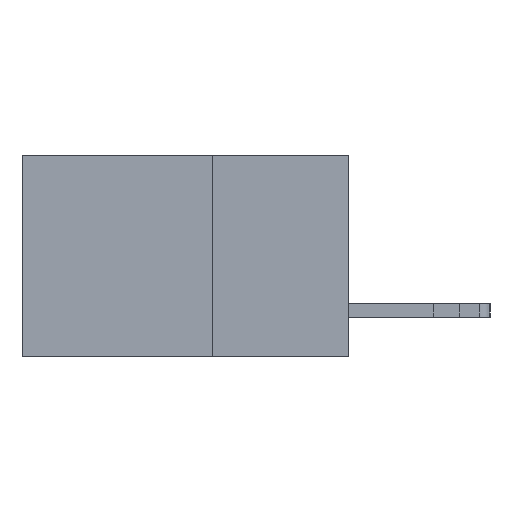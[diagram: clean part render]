
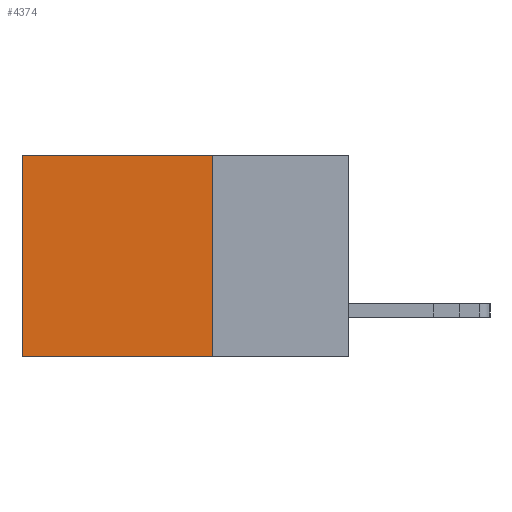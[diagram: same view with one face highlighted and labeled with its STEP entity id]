
A CAD part, left-side view. The second image highlights one B-rep face of the part: STEP entity #4374.
In plain terms, the highlighted planar face has unit normal (-1, 0, 0).
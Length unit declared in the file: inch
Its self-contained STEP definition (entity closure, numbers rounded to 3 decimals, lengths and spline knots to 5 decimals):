
#1281 = LINE ( 'NONE', #13152, #12820 ) ;
#1387 = DIRECTION ( 'NONE',  ( 0., 0., -1. ) ) ;
#1881 = VECTOR ( 'NONE', #18855, 39.37008 ) ;
#2364 = LINE ( 'NONE', #11405, #1881 ) ;
#2693 = VERTEX_POINT ( 'NONE', #4272 ) ;
#2909 = CARTESIAN_POINT ( 'NONE',  ( 0.298, 0.25, 0. ) ) ;
#4272 = CARTESIAN_POINT ( 'NONE',  ( 0.298, 0.25, -0.37 ) ) ;
#4374 = ADVANCED_FACE ( 'NONE', ( #13773 ), #11928, .F. ) ;
#4414 = DIRECTION ( 'NONE',  ( 1., 0., 0. ) ) ;
#4435 = EDGE_LOOP ( 'NONE', ( #9467, #10692, #15013, #9025 ) ) ;
#4733 = EDGE_CURVE ( 'NONE', #7990, #11289, #11190, .T. ) ;
#4887 = EDGE_CURVE ( 'NONE', #10564, #7990, #1281, .T. ) ;
#5282 = LINE ( 'NONE', #10419, #16817 ) ;
#7990 = VERTEX_POINT ( 'NONE', #11237 ) ;
#9025 = ORIENTED_EDGE ( 'NONE', *, *, #4887, .T. ) ;
#9467 = ORIENTED_EDGE ( 'NONE', *, *, #4733, .T. ) ;
#9555 = CARTESIAN_POINT ( 'NONE',  ( 0.298, 0.25, 0. ) ) ;
#9861 = DIRECTION ( 'NONE',  ( 0., 0., -1. ) ) ;
#10419 = CARTESIAN_POINT ( 'NONE',  ( 0.298, 0.25, 0. ) ) ;
#10564 = VERTEX_POINT ( 'NONE', #9555 ) ;
#10692 = ORIENTED_EDGE ( 'NONE', *, *, #18656, .F. ) ;
#11190 = LINE ( 'NONE', #14215, #14708 ) ;
#11237 = CARTESIAN_POINT ( 'NONE',  ( 0.298, 0.6, 0. ) ) ;
#11289 = VERTEX_POINT ( 'NONE', #18541 ) ;
#11405 = CARTESIAN_POINT ( 'NONE',  ( 0.298, 0.25, -0.37 ) ) ;
#11928 = PLANE ( 'NONE',  #13498 ) ;
#12820 = VECTOR ( 'NONE', #16102, 39.37008 ) ;
#13152 = CARTESIAN_POINT ( 'NONE',  ( 0.298, 0.25, 0. ) ) ;
#13498 = AXIS2_PLACEMENT_3D ( 'NONE', #2909, #4414, #14943 ) ;
#13773 = FACE_OUTER_BOUND ( 'NONE', #4435, .T. ) ;
#14215 = CARTESIAN_POINT ( 'NONE',  ( 0.298, 0.6, 0. ) ) ;
#14708 = VECTOR ( 'NONE', #9861, 39.37008 ) ;
#14943 = DIRECTION ( 'NONE',  ( 0., 0., -1. ) ) ;
#15013 = ORIENTED_EDGE ( 'NONE', *, *, #16574, .F. ) ;
#16102 = DIRECTION ( 'NONE',  ( 0., 1., 0. ) ) ;
#16574 = EDGE_CURVE ( 'NONE', #10564, #2693, #5282, .T. ) ;
#16817 = VECTOR ( 'NONE', #1387, 39.37008 ) ;
#18541 = CARTESIAN_POINT ( 'NONE',  ( 0.298, 0.6, -0.37 ) ) ;
#18656 = EDGE_CURVE ( 'NONE', #2693, #11289, #2364, .T. ) ;
#18855 = DIRECTION ( 'NONE',  ( 0., 1., 0. ) ) ;
